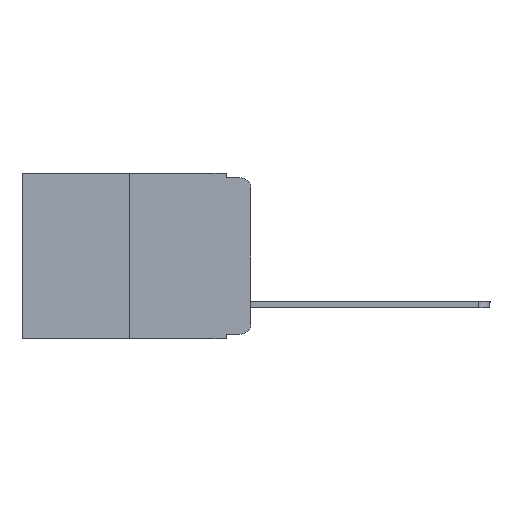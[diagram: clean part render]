
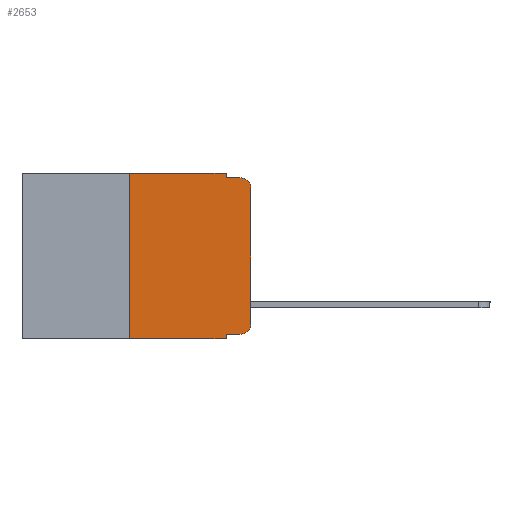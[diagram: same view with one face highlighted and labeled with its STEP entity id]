
A CAD part, left-side view. The second image highlights one B-rep face of the part: STEP entity #2653.
In plain terms, the highlighted planar face has unit normal (-1, 0, 0).
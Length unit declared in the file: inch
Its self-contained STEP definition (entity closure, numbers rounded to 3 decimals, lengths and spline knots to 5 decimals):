
#523 = EDGE_CURVE ( 'NONE', #9833, #17381, #8634, .T. ) ;
#940 = DIRECTION ( 'NONE',  ( 0., -1., 0. ) ) ;
#975 = CARTESIAN_POINT ( 'NONE',  ( 0., 0., 0. ) ) ;
#1038 = CARTESIAN_POINT ( 'NONE',  ( 0., 0.473, -0.343 ) ) ;
#1270 = ORIENTED_EDGE ( 'NONE', *, *, #11313, .T. ) ;
#1648 = CARTESIAN_POINT ( 'NONE',  ( 0., 0.051, 0. ) ) ;
#1985 = VECTOR ( 'NONE', #17779, 39.37008 ) ;
#2041 = LINE ( 'NONE', #6729, #10060 ) ;
#2042 = EDGE_CURVE ( 'NONE', #10653, #9537, #20454, .T. ) ;
#2497 = AXIS2_PLACEMENT_3D ( 'NONE', #10264, #13671, #2960 ) ;
#2623 = VECTOR ( 'NONE', #13692, 39.37008 ) ;
#2653 = ADVANCED_FACE ( 'NONE', ( #12619 ), #18846, .F. ) ;
#2960 = DIRECTION ( 'NONE',  ( 0., 0., -1. ) ) ;
#3155 = AXIS2_PLACEMENT_3D ( 'NONE', #4772, #19139, #17684 ) ;
#3238 = EDGE_CURVE ( 'NONE', #3759, #9975, #16411, .T. ) ;
#3759 = VERTEX_POINT ( 'NONE', #3782 ) ;
#3782 = CARTESIAN_POINT ( 'NONE',  ( 0., 0.051, -0.01 ) ) ;
#3867 = CARTESIAN_POINT ( 'NONE',  ( 0., 0.051, -0.333 ) ) ;
#4231 = LINE ( 'NONE', #18389, #2623 ) ;
#4589 = CARTESIAN_POINT ( 'NONE',  ( 0., 0.473, 0. ) ) ;
#4772 = CARTESIAN_POINT ( 'NONE',  ( 0., 0.02, -0.03 ) ) ;
#4893 = EDGE_CURVE ( 'NONE', #9194, #7855, #14946, .T. ) ;
#5230 = ORIENTED_EDGE ( 'NONE', *, *, #8796, .T. ) ;
#6228 = EDGE_CURVE ( 'NONE', #14519, #7855, #19176, .T. ) ;
#6652 = LINE ( 'NONE', #17769, #10680 ) ;
#6729 = CARTESIAN_POINT ( 'NONE',  ( 0., 0.051, -0.333 ) ) ;
#7471 = ORIENTED_EDGE ( 'NONE', *, *, #3238, .F. ) ;
#7699 = ORIENTED_EDGE ( 'NONE', *, *, #523, .F. ) ;
#7817 = CIRCLE ( 'NONE', #3155, 0.02 ) ;
#7853 = ORIENTED_EDGE ( 'NONE', *, *, #14051, .T. ) ;
#7855 = VERTEX_POINT ( 'NONE', #14660 ) ;
#8186 = EDGE_CURVE ( 'NONE', #14519, #9833, #6652, .T. ) ;
#8310 = CARTESIAN_POINT ( 'NONE',  ( 0., 0.051, 0. ) ) ;
#8328 = ORIENTED_EDGE ( 'NONE', *, *, #20294, .F. ) ;
#8634 = LINE ( 'NONE', #19347, #1985 ) ;
#8694 = DIRECTION ( 'NONE',  ( 0., 0., 1. ) ) ;
#8796 = EDGE_CURVE ( 'NONE', #9537, #14846, #17946, .T. ) ;
#9194 = VERTEX_POINT ( 'NONE', #3867 ) ;
#9276 = VECTOR ( 'NONE', #16609, 39.37008 ) ;
#9504 = DIRECTION ( 'NONE',  ( 1., 0., 0. ) ) ;
#9537 = VERTEX_POINT ( 'NONE', #13213 ) ;
#9833 = VERTEX_POINT ( 'NONE', #16195 ) ;
#9975 = VERTEX_POINT ( 'NONE', #13789 ) ;
#10060 = VECTOR ( 'NONE', #14315, 39.37008 ) ;
#10072 = DIRECTION ( 'NONE',  ( 0., 0., 1. ) ) ;
#10264 = CARTESIAN_POINT ( 'NONE',  ( 0., 0.02, -0.313 ) ) ;
#10653 = VERTEX_POINT ( 'NONE', #13511 ) ;
#10680 = VECTOR ( 'NONE', #10072, 39.37008 ) ;
#11313 = EDGE_CURVE ( 'NONE', #9194, #10653, #2041, .T. ) ;
#12619 = FACE_OUTER_BOUND ( 'NONE', #16535, .T. ) ;
#13213 = CARTESIAN_POINT ( 'NONE',  ( 0., 0., -0.313 ) ) ;
#13511 = CARTESIAN_POINT ( 'NONE',  ( 0., 0.02, -0.333 ) ) ;
#13671 = DIRECTION ( 'NONE',  ( -1., 0., 0. ) ) ;
#13692 = DIRECTION ( 'NONE',  ( 0., 0., -1. ) ) ;
#13747 = ORIENTED_EDGE ( 'NONE', *, *, #2042, .T. ) ;
#13789 = CARTESIAN_POINT ( 'NONE',  ( 0., 0.02, -0.01 ) ) ;
#14051 = EDGE_CURVE ( 'NONE', #14846, #9975, #7817, .T. ) ;
#14315 = DIRECTION ( 'NONE',  ( 0., -1., 0. ) ) ;
#14519 = VERTEX_POINT ( 'NONE', #16608 ) ;
#14660 = CARTESIAN_POINT ( 'NONE',  ( 0., 0.051, -0.343 ) ) ;
#14846 = VERTEX_POINT ( 'NONE', #17638 ) ;
#14946 = LINE ( 'NONE', #8310, #16771 ) ;
#15315 = ORIENTED_EDGE ( 'NONE', *, *, #6228, .T. ) ;
#15920 = AXIS2_PLACEMENT_3D ( 'NONE', #4589, #9504, #15953 ) ;
#15953 = DIRECTION ( 'NONE',  ( 0., 0., -1. ) ) ;
#16195 = CARTESIAN_POINT ( 'NONE',  ( 0., 0.25, 0. ) ) ;
#16329 = VECTOR ( 'NONE', #8694, 39.37008 ) ;
#16411 = LINE ( 'NONE', #19725, #9276 ) ;
#16535 = EDGE_LOOP ( 'NONE', ( #5230, #7853, #7471, #8328, #7699, #19916, #15315, #18636, #1270, #13747 ) ) ;
#16609 = DIRECTION ( 'NONE',  ( 0., -1., 0. ) ) ;
#16608 = CARTESIAN_POINT ( 'NONE',  ( 0., 0.25, -0.343 ) ) ;
#16771 = VECTOR ( 'NONE', #18169, 39.37008 ) ;
#17381 = VERTEX_POINT ( 'NONE', #1648 ) ;
#17638 = CARTESIAN_POINT ( 'NONE',  ( 0., 0., -0.03 ) ) ;
#17684 = DIRECTION ( 'NONE',  ( 0., 0., -1. ) ) ;
#17769 = CARTESIAN_POINT ( 'NONE',  ( 0., 0.25, 0. ) ) ;
#17779 = DIRECTION ( 'NONE',  ( 0., -1., 0. ) ) ;
#17946 = LINE ( 'NONE', #975, #16329 ) ;
#18169 = DIRECTION ( 'NONE',  ( 0., 0., -1. ) ) ;
#18389 = CARTESIAN_POINT ( 'NONE',  ( 0., 0.051, 0. ) ) ;
#18636 = ORIENTED_EDGE ( 'NONE', *, *, #4893, .F. ) ;
#18846 = PLANE ( 'NONE',  #15920 ) ;
#19139 = DIRECTION ( 'NONE',  ( -1., 0., 0. ) ) ;
#19176 = LINE ( 'NONE', #1038, #20584 ) ;
#19347 = CARTESIAN_POINT ( 'NONE',  ( 0., 0.473, 0. ) ) ;
#19725 = CARTESIAN_POINT ( 'NONE',  ( 0., 0.051, -0.01 ) ) ;
#19916 = ORIENTED_EDGE ( 'NONE', *, *, #8186, .F. ) ;
#20294 = EDGE_CURVE ( 'NONE', #17381, #3759, #4231, .T. ) ;
#20454 = CIRCLE ( 'NONE', #2497, 0.02 ) ;
#20584 = VECTOR ( 'NONE', #940, 39.37008 ) ;
